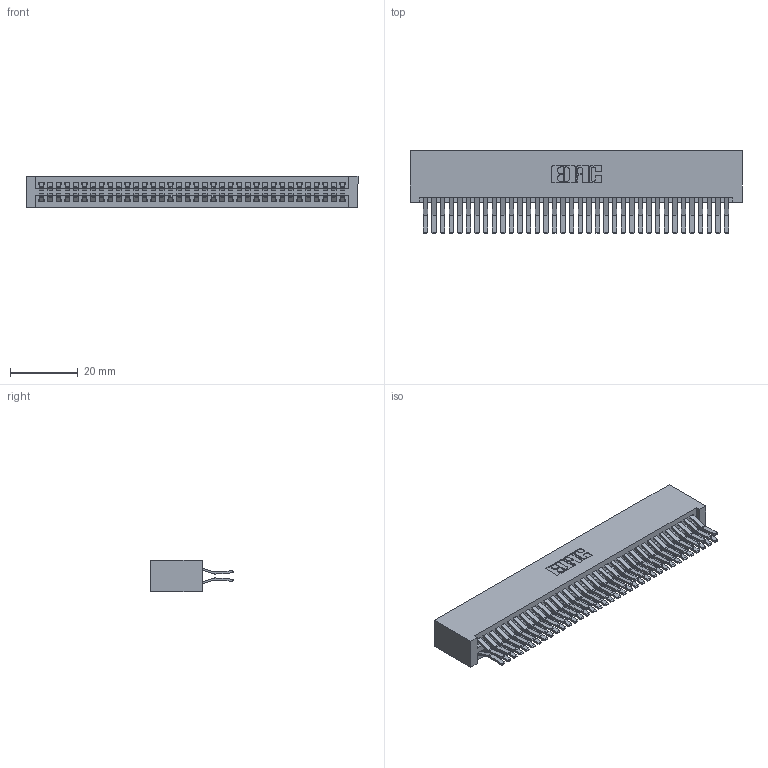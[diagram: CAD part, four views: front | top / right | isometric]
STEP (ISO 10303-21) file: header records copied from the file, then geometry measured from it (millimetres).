
FILE_DESCRIPTION (( 'STEP AP203' ), '1' );
FILE_NAME ('345-072-560-201.STEP', '2019-10-31T05:06:26', ( '' ), ( '' ), 'SwSTEP 2.0', 'SolidWorks 2016', '' );
FILE_SCHEMA (( 'CONFIG_CONTROL_DESIGN' ));
Length unit declared in the file: inch
Products named in the file (3): 345-292-001_560 Tail; 345-072-560-201; 345 Part_No Mounting Lugs
Assembly tree (73 placements, depth 2):
  345-072-560-201
    345 Part_No Mounting Lugs
    345-292-001_560 Tail  x72
Bounding box: 98.04 x 24.45 x 9.4 mm (x, y, z)
Volume: 10556.2 mm3; surface area: 17004.7 mm2
Topology: 73 solids, 73 shells, 3862 faces, 11477 edges, 7554 vertices
Faces by surface type: plane 2452, cylinder 1410
Entity records: 28865 total; most frequent: CARTESIAN_POINT 4844, ORIENTED_EDGE 4778, DIRECTION 4277, EDGE_CURVE 2389, LINE 2117, VECTOR 2117, VERTEX_POINT 1590, AXIS2_PLACEMENT_3D 1080
